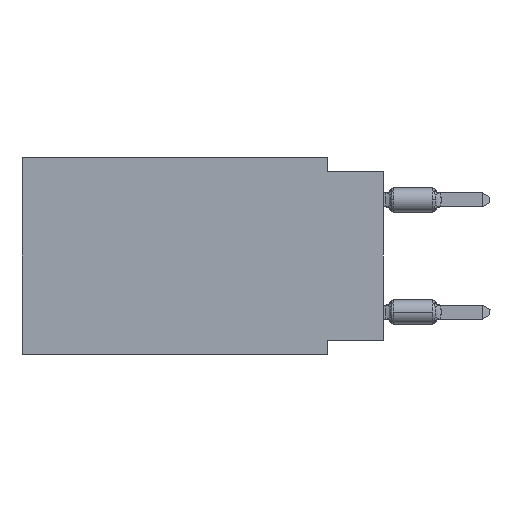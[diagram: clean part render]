
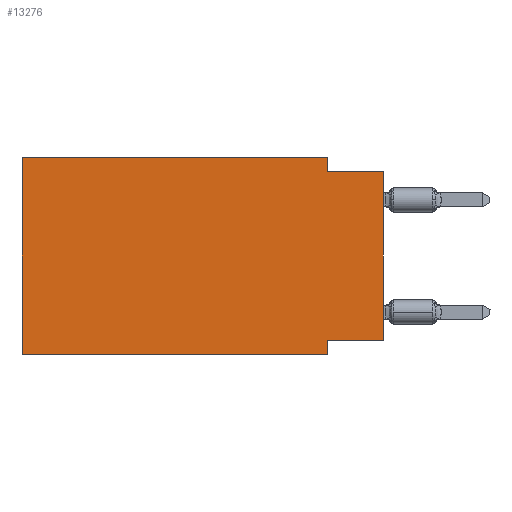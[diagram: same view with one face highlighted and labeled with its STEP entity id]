
A CAD part, left-side view. The second image highlights one B-rep face of the part: STEP entity #13276.
In plain terms, the highlighted planar face has unit normal (-1, 0, 0).
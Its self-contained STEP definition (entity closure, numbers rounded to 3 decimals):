
#1650 = EDGE_CURVE ( 'NONE', #27628, #11232, #11125, .T. ) ;
#3678 = VECTOR ( 'NONE', #43074, 1000. ) ;
#4768 = LINE ( 'NONE', #37556, #10746 ) ;
#6522 = CARTESIAN_POINT ( 'NONE',  ( 0., 2.54, 0. ) ) ;
#6935 = VECTOR ( 'NONE', #15424, 1000. ) ;
#7199 = EDGE_CURVE ( 'NONE', #60153, #19382, #4768, .T. ) ;
#10657 = ORIENTED_EDGE ( 'NONE', *, *, #23470, .F. ) ;
#10746 = VECTOR ( 'NONE', #70012, 1000. ) ;
#11125 = LINE ( 'NONE', #43215, #6935 ) ;
#11232 = VERTEX_POINT ( 'NONE', #22963 ) ;
#11701 = FACE_OUTER_BOUND ( 'NONE', #33632, .T. ) ;
#12525 = CARTESIAN_POINT ( 'NONE',  ( 0., 2.54, -0.635 ) ) ;
#12543 = CARTESIAN_POINT ( 'NONE',  ( 0., 16.383, -8.89 ) ) ;
#13276 = ADVANCED_FACE ( 'NONE', ( #11701 ), #13349, .F. ) ;
#13349 = PLANE ( 'NONE',  #14541 ) ;
#14541 = AXIS2_PLACEMENT_3D ( 'NONE', #57550, #68582, #29761 ) ;
#14923 = EDGE_CURVE ( 'NONE', #16169, #16288, #19634, .T. ) ;
#15424 = DIRECTION ( 'NONE',  ( 0., 0., 1. ) ) ;
#16169 = VERTEX_POINT ( 'NONE', #52446 ) ;
#16288 = VERTEX_POINT ( 'NONE', #38148 ) ;
#17336 = ORIENTED_EDGE ( 'NONE', *, *, #29375, .F. ) ;
#19382 = VERTEX_POINT ( 'NONE', #12525 ) ;
#19634 = LINE ( 'NONE', #19981, #56980 ) ;
#19981 = CARTESIAN_POINT ( 'NONE',  ( 0., 0., 0. ) ) ;
#20453 = CARTESIAN_POINT ( 'NONE',  ( 0., 16.383, 0. ) ) ;
#20850 = CARTESIAN_POINT ( 'NONE',  ( 0., 2.54, -8.255 ) ) ;
#22963 = CARTESIAN_POINT ( 'NONE',  ( 0., 16.383, 0. ) ) ;
#23234 = CARTESIAN_POINT ( 'NONE',  ( 0., 0., -0.635 ) ) ;
#23470 = EDGE_CURVE ( 'NONE', #67846, #47254, #60178, .T. ) ;
#27628 = VERTEX_POINT ( 'NONE', #12543 ) ;
#28621 = EDGE_CURVE ( 'NONE', #19382, #16288, #45322, .T. ) ;
#29375 = EDGE_CURVE ( 'NONE', #16169, #67846, #43400, .T. ) ;
#29689 = ORIENTED_EDGE ( 'NONE', *, *, #58344, .F. ) ;
#29761 = DIRECTION ( 'NONE',  ( 0., 0., -1. ) ) ;
#32709 = CARTESIAN_POINT ( 'NONE',  ( 0., 0., -8.255 ) ) ;
#32731 = VECTOR ( 'NONE', #49805, 1000. ) ;
#32821 = VECTOR ( 'NONE', #40556, 1000. ) ;
#33632 = EDGE_LOOP ( 'NONE', ( #40397, #42903, #62153, #29689, #70332, #36390, #10657, #17336 ) ) ;
#36390 = ORIENTED_EDGE ( 'NONE', *, *, #64991, .T. ) ;
#37556 = CARTESIAN_POINT ( 'NONE',  ( 0., 2.54, 0. ) ) ;
#38148 = CARTESIAN_POINT ( 'NONE',  ( 0., 0., -0.635 ) ) ;
#40397 = ORIENTED_EDGE ( 'NONE', *, *, #14923, .T. ) ;
#40556 = DIRECTION ( 'NONE',  ( 0., -1., 0. ) ) ;
#41020 = DIRECTION ( 'NONE',  ( 0., 0., 1. ) ) ;
#41616 = CARTESIAN_POINT ( 'NONE',  ( 0., 16.383, -8.89 ) ) ;
#42903 = ORIENTED_EDGE ( 'NONE', *, *, #28621, .F. ) ;
#43074 = DIRECTION ( 'NONE',  ( 0., 0., -1. ) ) ;
#43215 = CARTESIAN_POINT ( 'NONE',  ( 0., 16.383, 0. ) ) ;
#43400 = LINE ( 'NONE', #32709, #32731 ) ;
#45322 = LINE ( 'NONE', #23234, #55382 ) ;
#47254 = VERTEX_POINT ( 'NONE', #52626 ) ;
#49805 = DIRECTION ( 'NONE',  ( 0., 1., 0. ) ) ;
#50547 = VECTOR ( 'NONE', #64301, 1000. ) ;
#52446 = CARTESIAN_POINT ( 'NONE',  ( 0., 0., -8.255 ) ) ;
#52626 = CARTESIAN_POINT ( 'NONE',  ( 0., 2.54, -8.89 ) ) ;
#55382 = VECTOR ( 'NONE', #60665, 1000. ) ;
#56622 = LINE ( 'NONE', #41616, #32821 ) ;
#56980 = VECTOR ( 'NONE', #41020, 1000. ) ;
#57550 = CARTESIAN_POINT ( 'NONE',  ( 0., 16.383, 0. ) ) ;
#58238 = LINE ( 'NONE', #20453, #50547 ) ;
#58344 = EDGE_CURVE ( 'NONE', #11232, #60153, #58238, .T. ) ;
#60153 = VERTEX_POINT ( 'NONE', #6522 ) ;
#60178 = LINE ( 'NONE', #70510, #3678 ) ;
#60665 = DIRECTION ( 'NONE',  ( 0., -1., 0. ) ) ;
#62153 = ORIENTED_EDGE ( 'NONE', *, *, #7199, .F. ) ;
#64301 = DIRECTION ( 'NONE',  ( 0., -1., 0. ) ) ;
#64991 = EDGE_CURVE ( 'NONE', #27628, #47254, #56622, .T. ) ;
#67846 = VERTEX_POINT ( 'NONE', #20850 ) ;
#68582 = DIRECTION ( 'NONE',  ( 1., 0., 0. ) ) ;
#70012 = DIRECTION ( 'NONE',  ( 0., 0., -1. ) ) ;
#70332 = ORIENTED_EDGE ( 'NONE', *, *, #1650, .F. ) ;
#70510 = CARTESIAN_POINT ( 'NONE',  ( 0., 2.54, -8.89 ) ) ;
